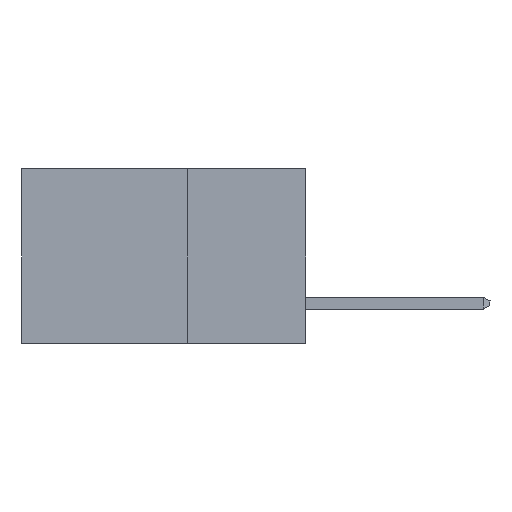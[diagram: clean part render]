
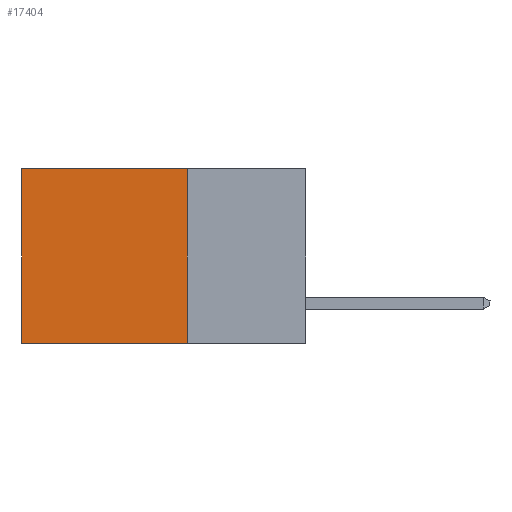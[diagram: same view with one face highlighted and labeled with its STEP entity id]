
A CAD part, left-side view. The second image highlights one B-rep face of the part: STEP entity #17404.
In plain terms, the highlighted planar face has unit normal (-1, 0, 0).
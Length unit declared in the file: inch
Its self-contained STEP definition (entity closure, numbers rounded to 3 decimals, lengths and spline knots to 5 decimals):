
#713 = DIRECTION ( 'NONE',  ( 0., 1., 0. ) ) ;
#777 = VERTEX_POINT ( 'NONE', #18629 ) ;
#805 = EDGE_CURVE ( 'NONE', #8091, #4303, #15554, .T. ) ;
#1422 = VERTEX_POINT ( 'NONE', #14142 ) ;
#2211 = DIRECTION ( 'NONE',  ( 0., 0., -1. ) ) ;
#2214 = ORIENTED_EDGE ( 'NONE', *, *, #3737, .T. ) ;
#3737 = EDGE_CURVE ( 'NONE', #8091, #1422, #12169, .T. ) ;
#3915 = PLANE ( 'NONE',  #11222 ) ;
#4303 = VERTEX_POINT ( 'NONE', #17536 ) ;
#4806 = EDGE_CURVE ( 'NONE', #1422, #777, #13266, .T. ) ;
#5532 = VECTOR ( 'NONE', #713, 39.37008 ) ;
#7304 = CARTESIAN_POINT ( 'NONE',  ( 0.2615, 0.25, -0.37 ) ) ;
#7417 = VECTOR ( 'NONE', #12146, 39.37008 ) ;
#8091 = VERTEX_POINT ( 'NONE', #9799 ) ;
#8238 = VECTOR ( 'NONE', #13045, 39.37008 ) ;
#8429 = CARTESIAN_POINT ( 'NONE',  ( 0.2615, 0.25, -0.37 ) ) ;
#8544 = CARTESIAN_POINT ( 'NONE',  ( 0.2615, 0.6, -0.37 ) ) ;
#8774 = VECTOR ( 'NONE', #13367, 39.37008 ) ;
#9799 = CARTESIAN_POINT ( 'NONE',  ( 0.2615, 0.25, 0. ) ) ;
#10041 = LINE ( 'NONE', #8429, #8774 ) ;
#10765 = CARTESIAN_POINT ( 'NONE',  ( 0.2615, 0.25, 0. ) ) ;
#11222 = AXIS2_PLACEMENT_3D ( 'NONE', #18437, #20253, #2211 ) ;
#11349 = ORIENTED_EDGE ( 'NONE', *, *, #805, .F. ) ;
#11973 = EDGE_CURVE ( 'NONE', #4303, #777, #10041, .T. ) ;
#12043 = EDGE_LOOP ( 'NONE', ( #19484, #18364, #11349, #2214 ) ) ;
#12146 = DIRECTION ( 'NONE',  ( 0., 0., -1. ) ) ;
#12169 = LINE ( 'NONE', #10765, #5532 ) ;
#13045 = DIRECTION ( 'NONE',  ( 0., 0., -1. ) ) ;
#13266 = LINE ( 'NONE', #8544, #8238 ) ;
#13367 = DIRECTION ( 'NONE',  ( 0., 1., 0. ) ) ;
#14142 = CARTESIAN_POINT ( 'NONE',  ( 0.2615, 0.6, 0. ) ) ;
#15554 = LINE ( 'NONE', #7304, #7417 ) ;
#17404 = ADVANCED_FACE ( 'NONE', ( #18651 ), #3915, .F. ) ;
#17536 = CARTESIAN_POINT ( 'NONE',  ( 0.2615, 0.25, -0.37 ) ) ;
#18364 = ORIENTED_EDGE ( 'NONE', *, *, #11973, .F. ) ;
#18437 = CARTESIAN_POINT ( 'NONE',  ( 0.2615, 0.25, -0.37 ) ) ;
#18629 = CARTESIAN_POINT ( 'NONE',  ( 0.2615, 0.6, -0.37 ) ) ;
#18651 = FACE_OUTER_BOUND ( 'NONE', #12043, .T. ) ;
#19484 = ORIENTED_EDGE ( 'NONE', *, *, #4806, .T. ) ;
#20253 = DIRECTION ( 'NONE',  ( 1., 0., 0. ) ) ;
